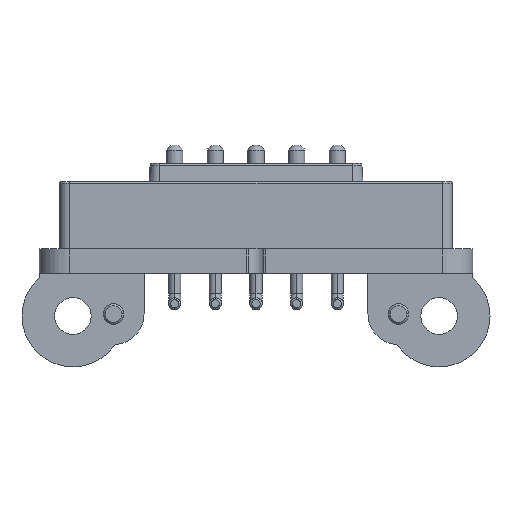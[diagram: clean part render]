
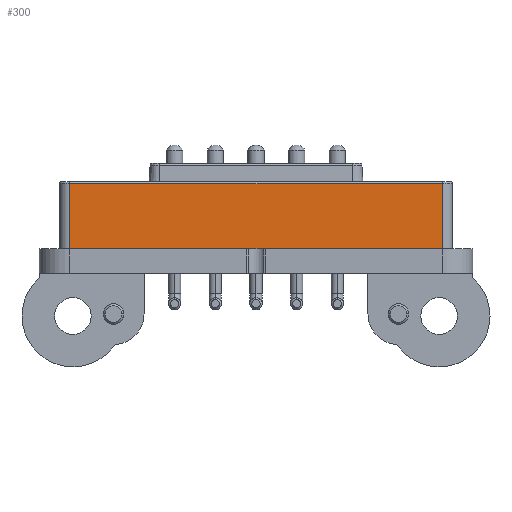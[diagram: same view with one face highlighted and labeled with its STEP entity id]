
A CAD part, front view. The second image highlights one B-rep face of the part: STEP entity #300.
In plain terms, the highlighted planar face has unit normal (0, -1, 0).
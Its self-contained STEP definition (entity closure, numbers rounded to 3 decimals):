
#165 = VECTOR ( 'NONE', #6305, 1000. ) ;
#300 = ADVANCED_FACE ( 'NONE', ( #3030 ), #7821, .F. ) ;
#1825 = LINE ( 'NONE', #6373, #165 ) ;
#2018 = CARTESIAN_POINT ( 'NONE',  ( -9.15, -2.5, -3.3 ) ) ;
#3030 = FACE_OUTER_BOUND ( 'NONE', #6484, .T. ) ;
#3355 = EDGE_CURVE ( 'NONE', #12767, #11004, #1825, .T. ) ;
#3594 = LINE ( 'NONE', #10293, #9455 ) ;
#4395 = ORIENTED_EDGE ( 'NONE', *, *, #3355, .T. ) ;
#4407 = CARTESIAN_POINT ( 'NONE',  ( -9.15, -2.5, -0.1 ) ) ;
#5559 = DIRECTION ( 'NONE',  ( 0., 1., 0. ) ) ;
#6305 = DIRECTION ( 'NONE',  ( 1., 0., 0. ) ) ;
#6373 = CARTESIAN_POINT ( 'NONE',  ( -9.15, -2.5, -3.3 ) ) ;
#6463 = DIRECTION ( 'NONE',  ( -1., 0., 0. ) ) ;
#6484 = EDGE_LOOP ( 'NONE', ( #13479, #4395, #12808, #13694 ) ) ;
#7355 = VERTEX_POINT ( 'NONE', #12484 ) ;
#7650 = DIRECTION ( 'NONE',  ( 0., 0., 1. ) ) ;
#7745 = LINE ( 'NONE', #12324, #12492 ) ;
#7821 = PLANE ( 'NONE',  #8172 ) ;
#8157 = DIRECTION ( 'NONE',  ( 0., 0., -1. ) ) ;
#8172 = AXIS2_PLACEMENT_3D ( 'NONE', #11207, #5559, #12393 ) ;
#8302 = EDGE_CURVE ( 'NONE', #7355, #13819, #7745, .T. ) ;
#8519 = EDGE_CURVE ( 'NONE', #11004, #7355, #12309, .T. ) ;
#9455 = VECTOR ( 'NONE', #8157, 1000. ) ;
#10293 = CARTESIAN_POINT ( 'NONE',  ( -9.15, -2.5, -0.1 ) ) ;
#10903 = CARTESIAN_POINT ( 'NONE',  ( 9.15, -2.5, -3.3 ) ) ;
#11004 = VERTEX_POINT ( 'NONE', #13859 ) ;
#11207 = CARTESIAN_POINT ( 'NONE',  ( 0., -2.5, -1.7 ) ) ;
#12309 = LINE ( 'NONE', #10903, #13143 ) ;
#12324 = CARTESIAN_POINT ( 'NONE',  ( 9.15, -2.5, -0.1 ) ) ;
#12367 = EDGE_CURVE ( 'NONE', #13819, #12767, #3594, .T. ) ;
#12393 = DIRECTION ( 'NONE',  ( 1., 0., 0. ) ) ;
#12484 = CARTESIAN_POINT ( 'NONE',  ( 9.15, -2.5, -0.1 ) ) ;
#12492 = VECTOR ( 'NONE', #6463, 1000. ) ;
#12767 = VERTEX_POINT ( 'NONE', #2018 ) ;
#12808 = ORIENTED_EDGE ( 'NONE', *, *, #8519, .T. ) ;
#13143 = VECTOR ( 'NONE', #7650, 1000. ) ;
#13479 = ORIENTED_EDGE ( 'NONE', *, *, #12367, .T. ) ;
#13694 = ORIENTED_EDGE ( 'NONE', *, *, #8302, .T. ) ;
#13819 = VERTEX_POINT ( 'NONE', #4407 ) ;
#13859 = CARTESIAN_POINT ( 'NONE',  ( 9.15, -2.5, -3.3 ) ) ;
